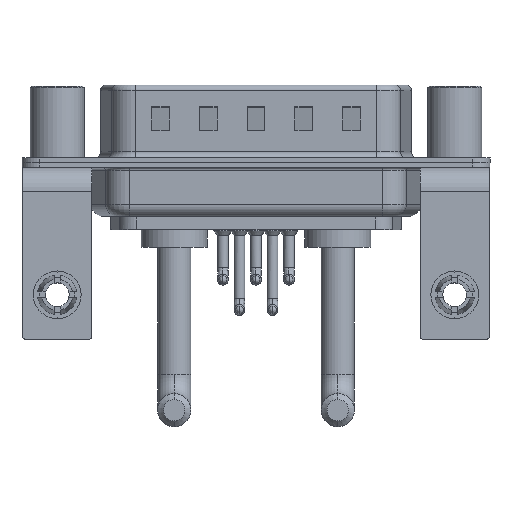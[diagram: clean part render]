
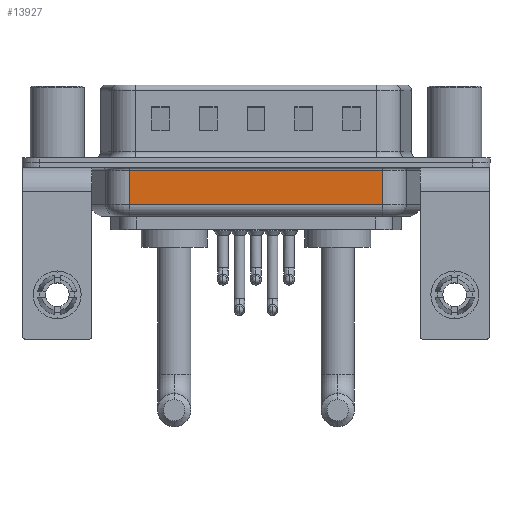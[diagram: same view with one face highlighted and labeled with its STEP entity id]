
A CAD part, front view. The second image highlights one B-rep face of the part: STEP entity #13927.
In plain terms, the highlighted planar face has unit normal (0, -1, 0).
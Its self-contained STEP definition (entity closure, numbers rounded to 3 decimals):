
#994 = VECTOR ( 'NONE', #14904, 1000. ) ;
#1361 = VECTOR ( 'NONE', #13394, 1000. ) ;
#1999 = CARTESIAN_POINT ( 'NONE',  ( 6.031, -5.35, -0.65 ) ) ;
#2512 = ORIENTED_EDGE ( 'NONE', *, *, #8469, .T. ) ;
#2721 = EDGE_CURVE ( 'NONE', #13953, #13971, #16753, .T. ) ;
#2736 = EDGE_CURVE ( 'NONE', #13953, #12740, #18874, .T. ) ;
#3288 = LINE ( 'NONE', #20378, #6521 ) ;
#3336 = EDGE_CURVE ( 'NONE', #17823, #13971, #9452, .T. ) ;
#4165 = VECTOR ( 'NONE', #9356, 1000. ) ;
#5509 = CARTESIAN_POINT ( 'NONE',  ( 6.031, -5.35, -3.5 ) ) ;
#6326 = EDGE_LOOP ( 'NONE', ( #23892, #9461, #2512, #21731 ) ) ;
#6521 = VECTOR ( 'NONE', #22344, 1000. ) ;
#7120 = CARTESIAN_POINT ( 'NONE',  ( 6.031, -5.35, -4.5 ) ) ;
#8469 = EDGE_CURVE ( 'NONE', #12740, #17823, #3288, .T. ) ;
#9356 = DIRECTION ( 'NONE',  ( 1., 0., 0. ) ) ;
#9452 = LINE ( 'NONE', #1999, #1361 ) ;
#9461 = ORIENTED_EDGE ( 'NONE', *, *, #2736, .T. ) ;
#9819 = AXIS2_PLACEMENT_3D ( 'NONE', #20091, #19732, #10335 ) ;
#10167 = CARTESIAN_POINT ( 'NONE',  ( 27.269, -5.35, -3.5 ) ) ;
#10335 = DIRECTION ( 'NONE',  ( 0., 0., 1. ) ) ;
#12422 = FACE_OUTER_BOUND ( 'NONE', #6326, .T. ) ;
#12740 = VERTEX_POINT ( 'NONE', #10167 ) ;
#12897 = CARTESIAN_POINT ( 'NONE',  ( 6.031, -5.35, -0.65 ) ) ;
#13394 = DIRECTION ( 'NONE',  ( -1., 0., 0. ) ) ;
#13927 = ADVANCED_FACE ( 'NONE', ( #12422 ), #14153, .F. ) ;
#13953 = VERTEX_POINT ( 'NONE', #19848 ) ;
#13971 = VERTEX_POINT ( 'NONE', #12897 ) ;
#14153 = PLANE ( 'NONE',  #9819 ) ;
#14904 = DIRECTION ( 'NONE',  ( 0., 0., 1. ) ) ;
#16039 = CARTESIAN_POINT ( 'NONE',  ( 27.269, -5.35, -0.65 ) ) ;
#16753 = LINE ( 'NONE', #7120, #994 ) ;
#17823 = VERTEX_POINT ( 'NONE', #16039 ) ;
#18874 = LINE ( 'NONE', #5509, #4165 ) ;
#19732 = DIRECTION ( 'NONE',  ( 0., 1., 0. ) ) ;
#19848 = CARTESIAN_POINT ( 'NONE',  ( 6.031, -5.35, -3.5 ) ) ;
#20091 = CARTESIAN_POINT ( 'NONE',  ( 6.031, -5.35, -4.5 ) ) ;
#20378 = CARTESIAN_POINT ( 'NONE',  ( 27.269, -5.35, -4.5 ) ) ;
#21731 = ORIENTED_EDGE ( 'NONE', *, *, #3336, .T. ) ;
#22344 = DIRECTION ( 'NONE',  ( 0., 0., 1. ) ) ;
#23892 = ORIENTED_EDGE ( 'NONE', *, *, #2721, .F. ) ;
